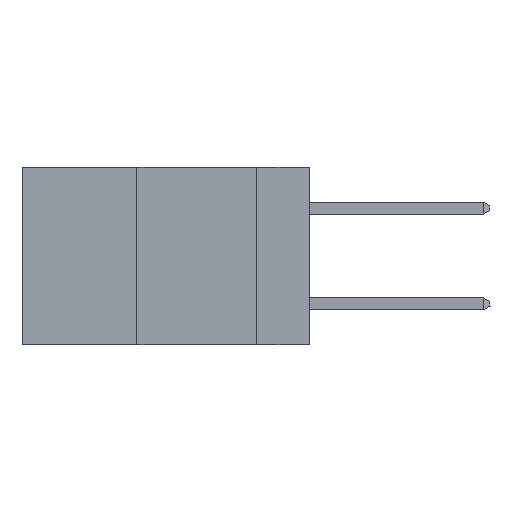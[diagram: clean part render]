
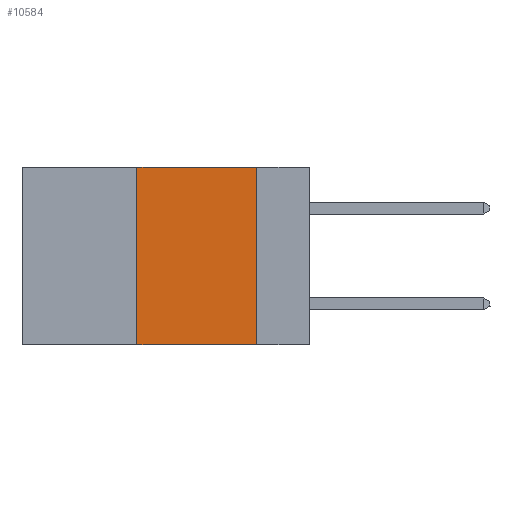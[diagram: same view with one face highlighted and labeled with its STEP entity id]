
A CAD part, left-side view. The second image highlights one B-rep face of the part: STEP entity #10584.
In plain terms, the highlighted planar face has unit normal (-1, 0, 0).
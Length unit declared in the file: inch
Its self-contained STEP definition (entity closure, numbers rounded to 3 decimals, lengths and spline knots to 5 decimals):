
#364 = LINE ( 'NONE', #1531, #5180 ) ;
#450 = ORIENTED_EDGE ( 'NONE', *, *, #8122, .F. ) ;
#984 = LINE ( 'NONE', #7164, #8018 ) ;
#1090 = DIRECTION ( 'NONE',  ( 1., 0., 0. ) ) ;
#1531 = CARTESIAN_POINT ( 'NONE',  ( 0., 0.6, 0. ) ) ;
#1538 = ORIENTED_EDGE ( 'NONE', *, *, #7086, .F. ) ;
#2088 = CARTESIAN_POINT ( 'NONE',  ( 0., 0.11, -0.37 ) ) ;
#2227 = VECTOR ( 'NONE', #6016, 39.37008 ) ;
#2532 = LINE ( 'NONE', #11553, #2227 ) ;
#3000 = VECTOR ( 'NONE', #6101, 39.37008 ) ;
#3942 = PLANE ( 'NONE',  #9603 ) ;
#4329 = DIRECTION ( 'NONE',  ( 0., 0., 1. ) ) ;
#4428 = DIRECTION ( 'NONE',  ( 0., -1., 0. ) ) ;
#5180 = VECTOR ( 'NONE', #4428, 39.37008 ) ;
#5479 = CARTESIAN_POINT ( 'NONE',  ( 0., 0.36, 0. ) ) ;
#5875 = EDGE_CURVE ( 'NONE', #11784, #6705, #984, .T. ) ;
#6016 = DIRECTION ( 'NONE',  ( 0., 0., -1. ) ) ;
#6101 = DIRECTION ( 'NONE',  ( 0., -1., 0. ) ) ;
#6619 = CARTESIAN_POINT ( 'NONE',  ( 0., 0.11, 0. ) ) ;
#6705 = VERTEX_POINT ( 'NONE', #5479 ) ;
#6828 = CARTESIAN_POINT ( 'NONE',  ( 0., 0.6, 0. ) ) ;
#6978 = CARTESIAN_POINT ( 'NONE',  ( 0., 0.36, -0.37 ) ) ;
#7086 = EDGE_CURVE ( 'NONE', #9481, #9665, #2532, .T. ) ;
#7164 = CARTESIAN_POINT ( 'NONE',  ( 0., 0.36, 0. ) ) ;
#7210 = EDGE_LOOP ( 'NONE', ( #1538, #450, #10108, #10017 ) ) ;
#7772 = LINE ( 'NONE', #11625, #3000 ) ;
#7783 = DIRECTION ( 'NONE',  ( 0., 0., -1. ) ) ;
#8018 = VECTOR ( 'NONE', #4329, 39.37008 ) ;
#8122 = EDGE_CURVE ( 'NONE', #6705, #9481, #364, .T. ) ;
#9481 = VERTEX_POINT ( 'NONE', #6619 ) ;
#9603 = AXIS2_PLACEMENT_3D ( 'NONE', #6828, #1090, #7783 ) ;
#9665 = VERTEX_POINT ( 'NONE', #2088 ) ;
#10017 = ORIENTED_EDGE ( 'NONE', *, *, #11834, .T. ) ;
#10108 = ORIENTED_EDGE ( 'NONE', *, *, #5875, .F. ) ;
#10584 = ADVANCED_FACE ( 'NONE', ( #11519 ), #3942, .F. ) ;
#11519 = FACE_OUTER_BOUND ( 'NONE', #7210, .T. ) ;
#11553 = CARTESIAN_POINT ( 'NONE',  ( 0., 0.11, 0. ) ) ;
#11625 = CARTESIAN_POINT ( 'NONE',  ( 0., 0.6, -0.37 ) ) ;
#11784 = VERTEX_POINT ( 'NONE', #6978 ) ;
#11834 = EDGE_CURVE ( 'NONE', #11784, #9665, #7772, .T. ) ;
